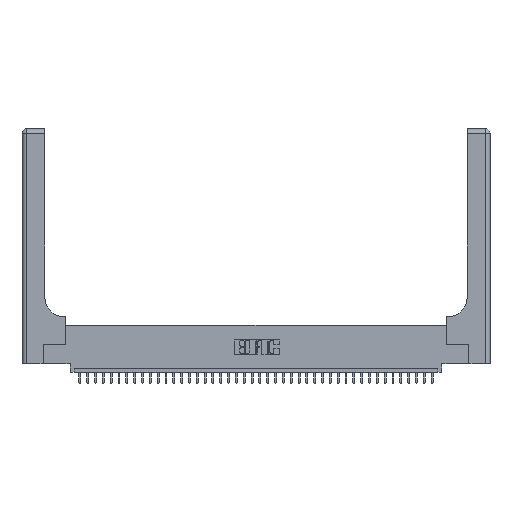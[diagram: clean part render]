
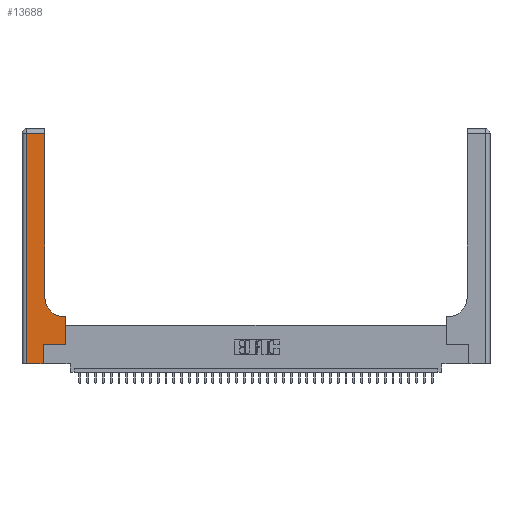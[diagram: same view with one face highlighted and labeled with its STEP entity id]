
A CAD part, top view. The second image highlights one B-rep face of the part: STEP entity #13688.
In plain terms, the highlighted planar face has unit normal (0, 0, 1).
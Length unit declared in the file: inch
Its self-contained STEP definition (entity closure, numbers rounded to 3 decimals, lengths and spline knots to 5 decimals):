
#1485 = VERTEX_POINT ( 'NONE', #31588 ) ;
#2299 = VECTOR ( 'NONE', #32496, 39.37008 ) ;
#2459 = EDGE_CURVE ( 'NONE', #35046, #38415, #31044, .T. ) ;
#2845 = CARTESIAN_POINT ( 'NONE',  ( 0.2915, 2.94, 0.37 ) ) ;
#3625 = ORIENTED_EDGE ( 'NONE', *, *, #10349, .T. ) ;
#3742 = DIRECTION ( 'NONE',  ( -1., 0., 0. ) ) ;
#4021 = LINE ( 'NONE', #32562, #26474 ) ;
#4293 = DIRECTION ( 'NONE',  ( 1., 0., 0. ) ) ;
#4309 = CARTESIAN_POINT ( 'NONE',  ( 0.269, 0.25, 0.37 ) ) ;
#4840 = EDGE_CURVE ( 'NONE', #14150, #22165, #4021, .T. ) ;
#5103 = CARTESIAN_POINT ( 'NONE',  ( 0.5585, 0.25, 0.37 ) ) ;
#6614 = VECTOR ( 'NONE', #15296, 39.37008 ) ;
#6664 = DIRECTION ( 'NONE',  ( 0., -1., 0. ) ) ;
#6719 = EDGE_LOOP ( 'NONE', ( #8913, #38981, #3625, #37789, #11566, #9355, #9250, #34901, #14946 ) ) ;
#6796 = CARTESIAN_POINT ( 'NONE',  ( 0.06, 3., 0.37 ) ) ;
#7999 = CARTESIAN_POINT ( 'NONE',  ( 0.5415, 0.85, 0.37 ) ) ;
#8110 = FACE_OUTER_BOUND ( 'NONE', #6719, .T. ) ;
#8130 = DIRECTION ( 'NONE',  ( 1., 0., 0. ) ) ;
#8913 = ORIENTED_EDGE ( 'NONE', *, *, #31222, .T. ) ;
#9250 = ORIENTED_EDGE ( 'NONE', *, *, #34180, .T. ) ;
#9355 = ORIENTED_EDGE ( 'NONE', *, *, #2459, .T. ) ;
#9371 = DIRECTION ( 'NONE',  ( -1., 0., 0. ) ) ;
#9398 = LINE ( 'NONE', #23210, #14266 ) ;
#9852 = VERTEX_POINT ( 'NONE', #36886 ) ;
#10349 = EDGE_CURVE ( 'NONE', #22165, #35241, #24148, .T. ) ;
#10941 = DIRECTION ( 'NONE',  ( -1., 0., 0. ) ) ;
#11255 = AXIS2_PLACEMENT_3D ( 'NONE', #33962, #22141, #3742 ) ;
#11265 = VECTOR ( 'NONE', #18352, 39.37008 ) ;
#11566 = ORIENTED_EDGE ( 'NONE', *, *, #31970, .T. ) ;
#11997 = AXIS2_PLACEMENT_3D ( 'NONE', #7999, #17217, #8130 ) ;
#13447 = EDGE_CURVE ( 'NONE', #22254, #23983, #18542, .T. ) ;
#13688 = ADVANCED_FACE ( 'NONE', ( #8110 ), #31062, .F. ) ;
#13924 = LINE ( 'NONE', #35856, #37168 ) ;
#14150 = VERTEX_POINT ( 'NONE', #2845 ) ;
#14266 = VECTOR ( 'NONE', #10941, 39.37008 ) ;
#14946 = ORIENTED_EDGE ( 'NONE', *, *, #13447, .T. ) ;
#15296 = DIRECTION ( 'NONE',  ( 0., 1., 0. ) ) ;
#16946 = CARTESIAN_POINT ( 'NONE',  ( 0., 0., 0.37 ) ) ;
#17217 = DIRECTION ( 'NONE',  ( 0., 0., -1. ) ) ;
#17636 = DIRECTION ( 'NONE',  ( 0., 1., 0. ) ) ;
#17648 = CARTESIAN_POINT ( 'NONE',  ( 0.06, 0., 0.37 ) ) ;
#18352 = DIRECTION ( 'NONE',  ( 0., 1., 0. ) ) ;
#18542 = CIRCLE ( 'NONE', #11997, 0.25 ) ;
#19627 = CARTESIAN_POINT ( 'NONE',  ( 0.269, 0.25, 0.37 ) ) ;
#22010 = CARTESIAN_POINT ( 'NONE',  ( 0.5415, 0.6, 0.37 ) ) ;
#22141 = DIRECTION ( 'NONE',  ( 0., 0., -1. ) ) ;
#22165 = VERTEX_POINT ( 'NONE', #37024 ) ;
#22254 = VERTEX_POINT ( 'NONE', #22010 ) ;
#23000 = VECTOR ( 'NONE', #4293, 39.37008 ) ;
#23210 = CARTESIAN_POINT ( 'NONE',  ( 0.2915, 0.6, 0.37 ) ) ;
#23311 = LINE ( 'NONE', #16946, #2299 ) ;
#23983 = VERTEX_POINT ( 'NONE', #37837 ) ;
#24148 = LINE ( 'NONE', #6796, #25538 ) ;
#25538 = VECTOR ( 'NONE', #6664, 39.37008 ) ;
#26474 = VECTOR ( 'NONE', #9371, 39.37008 ) ;
#29541 = LINE ( 'NONE', #30480, #6614 ) ;
#30480 = CARTESIAN_POINT ( 'NONE',  ( 0.269, 0., 0.37 ) ) ;
#31044 = LINE ( 'NONE', #19627, #23000 ) ;
#31062 = PLANE ( 'NONE',  #11255 ) ;
#31222 = EDGE_CURVE ( 'NONE', #23983, #14150, #13924, .T. ) ;
#31588 = CARTESIAN_POINT ( 'NONE',  ( 0.269, 0., 0.37 ) ) ;
#31970 = EDGE_CURVE ( 'NONE', #1485, #35046, #29541, .T. ) ;
#32496 = DIRECTION ( 'NONE',  ( 1., 0., 0. ) ) ;
#32562 = CARTESIAN_POINT ( 'NONE',  ( 0., 2.94, 0.37 ) ) ;
#33962 = CARTESIAN_POINT ( 'NONE',  ( 0., 3., 0.37 ) ) ;
#34180 = EDGE_CURVE ( 'NONE', #38415, #9852, #36004, .T. ) ;
#34901 = ORIENTED_EDGE ( 'NONE', *, *, #38997, .T. ) ;
#35046 = VERTEX_POINT ( 'NONE', #4309 ) ;
#35241 = VERTEX_POINT ( 'NONE', #17648 ) ;
#35856 = CARTESIAN_POINT ( 'NONE',  ( 0.2915, 3., 0.37 ) ) ;
#36004 = LINE ( 'NONE', #36810, #11265 ) ;
#36810 = CARTESIAN_POINT ( 'NONE',  ( 0.5585, 0.25, 0.37 ) ) ;
#36886 = CARTESIAN_POINT ( 'NONE',  ( 0.5585, 0.6, 0.37 ) ) ;
#37024 = CARTESIAN_POINT ( 'NONE',  ( 0.06, 2.94, 0.37 ) ) ;
#37168 = VECTOR ( 'NONE', #17636, 39.37008 ) ;
#37789 = ORIENTED_EDGE ( 'NONE', *, *, #38928, .T. ) ;
#37837 = CARTESIAN_POINT ( 'NONE',  ( 0.2915, 0.85, 0.37 ) ) ;
#38415 = VERTEX_POINT ( 'NONE', #5103 ) ;
#38928 = EDGE_CURVE ( 'NONE', #35241, #1485, #23311, .T. ) ;
#38981 = ORIENTED_EDGE ( 'NONE', *, *, #4840, .T. ) ;
#38997 = EDGE_CURVE ( 'NONE', #9852, #22254, #9398, .T. ) ;
